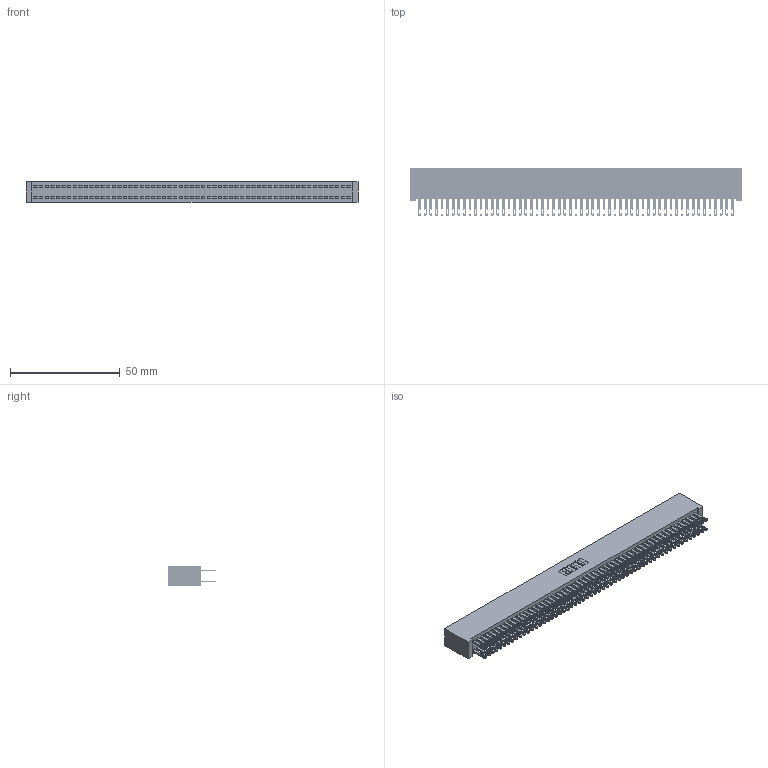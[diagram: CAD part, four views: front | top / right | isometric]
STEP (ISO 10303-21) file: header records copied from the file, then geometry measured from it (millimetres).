
FILE_DESCRIPTION (( 'STEP AP203' ), '1' );
FILE_NAME ('342-114-500-201.STEP', '2019-10-04T21:18:13', ( '' ), ( '' ), 'SwSTEP 2.0', 'SolidWorks 2016', '' );
FILE_SCHEMA (( 'CONFIG_CONTROL_DESIGN' ));
Length unit declared in the file: inch
Products named in the file (3): 342-114-500-201; 342 Part_Lugless; 345-292-001_345-293-100
Assembly tree (115 placements, depth 2):
  342-114-500-201
    342 Part_Lugless
    345-292-001_345-293-100  x114
Bounding box: 151.03 x 21.85 x 9.4 mm (x, y, z)
Volume: 14428.7 mm3; surface area: 25393.7 mm2
Topology: 115 solids, 115 shells, 5574 faces, 17033 edges, 11354 vertices
Faces by surface type: plane 3482, cylinder 2092
Entity records: 34251 total; most frequent: CARTESIAN_POINT 5654, ORIENTED_EDGE 5590, DIRECTION 4799, EDGE_CURVE 2795, LINE 2671, VECTOR 2671, VERTEX_POINT 1862, AXIS2_PLACEMENT_3D 1064
